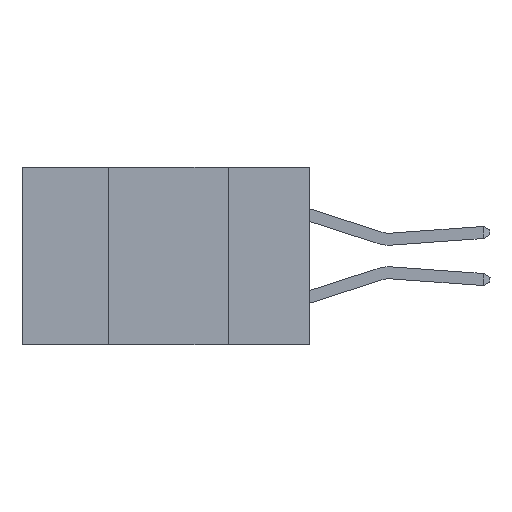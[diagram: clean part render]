
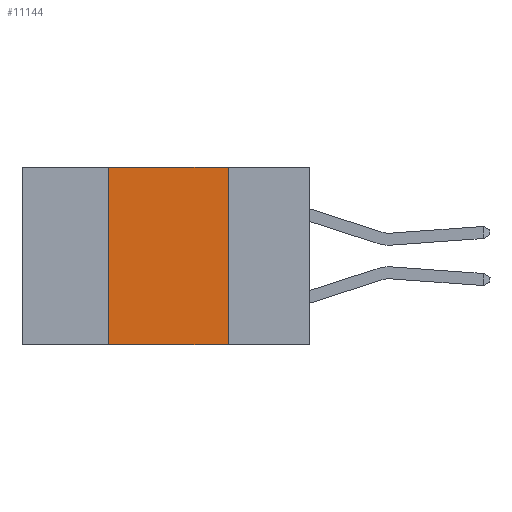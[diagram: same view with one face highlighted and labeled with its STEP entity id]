
A CAD part, left-side view. The second image highlights one B-rep face of the part: STEP entity #11144.
In plain terms, the highlighted planar face has unit normal (-1, 0, 0).
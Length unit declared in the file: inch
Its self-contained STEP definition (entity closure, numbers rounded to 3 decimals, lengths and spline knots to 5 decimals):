
#78 = VECTOR ( 'NONE', #6841, 39.37008 ) ;
#605 = CARTESIAN_POINT ( 'NONE',  ( 0., 0.17, 0. ) ) ;
#1331 = DIRECTION ( 'NONE',  ( 0., -1., 0. ) ) ;
#1500 = VERTEX_POINT ( 'NONE', #13177 ) ;
#1676 = LINE ( 'NONE', #15825, #78 ) ;
#2195 = CARTESIAN_POINT ( 'NONE',  ( 0., 0.6, 0. ) ) ;
#3289 = VERTEX_POINT ( 'NONE', #6100 ) ;
#3583 = VERTEX_POINT ( 'NONE', #18654 ) ;
#3704 = AXIS2_PLACEMENT_3D ( 'NONE', #2195, #12741, #5280 ) ;
#4783 = VERTEX_POINT ( 'NONE', #6198 ) ;
#5280 = DIRECTION ( 'NONE',  ( 0., 0., -1. ) ) ;
#6100 = CARTESIAN_POINT ( 'NONE',  ( 0., 0.17, 0. ) ) ;
#6198 = CARTESIAN_POINT ( 'NONE',  ( 0., 0.17, -0.37 ) ) ;
#6601 = EDGE_LOOP ( 'NONE', ( #7030, #7956, #11015, #7179 ) ) ;
#6708 = VECTOR ( 'NONE', #1331, 39.37008 ) ;
#6841 = DIRECTION ( 'NONE',  ( 0., -1., 0. ) ) ;
#6898 = PLANE ( 'NONE',  #3704 ) ;
#7030 = ORIENTED_EDGE ( 'NONE', *, *, #7323, .F. ) ;
#7179 = ORIENTED_EDGE ( 'NONE', *, *, #17079, .T. ) ;
#7323 = EDGE_CURVE ( 'NONE', #3289, #4783, #9662, .T. ) ;
#7956 = ORIENTED_EDGE ( 'NONE', *, *, #13563, .F. ) ;
#9662 = LINE ( 'NONE', #605, #12944 ) ;
#11015 = ORIENTED_EDGE ( 'NONE', *, *, #13642, .F. ) ;
#11074 = DIRECTION ( 'NONE',  ( 0., 0., -1. ) ) ;
#11144 = ADVANCED_FACE ( 'NONE', ( #18810 ), #6898, .F. ) ;
#11556 = CARTESIAN_POINT ( 'NONE',  ( 0., 0.42, 0. ) ) ;
#12741 = DIRECTION ( 'NONE',  ( 1., 0., 0. ) ) ;
#12944 = VECTOR ( 'NONE', #11074, 39.37008 ) ;
#13177 = CARTESIAN_POINT ( 'NONE',  ( 0., 0.42, 0. ) ) ;
#13563 = EDGE_CURVE ( 'NONE', #1500, #3289, #1676, .T. ) ;
#13642 = EDGE_CURVE ( 'NONE', #3583, #1500, #14933, .T. ) ;
#14933 = LINE ( 'NONE', #11556, #18398 ) ;
#15825 = CARTESIAN_POINT ( 'NONE',  ( 0., 0.6, 0. ) ) ;
#15863 = DIRECTION ( 'NONE',  ( 0., 0., 1. ) ) ;
#16328 = CARTESIAN_POINT ( 'NONE',  ( 0., 0.6, -0.37 ) ) ;
#17079 = EDGE_CURVE ( 'NONE', #3583, #4783, #18528, .T. ) ;
#18398 = VECTOR ( 'NONE', #15863, 39.37008 ) ;
#18528 = LINE ( 'NONE', #16328, #6708 ) ;
#18654 = CARTESIAN_POINT ( 'NONE',  ( 0., 0.42, -0.37 ) ) ;
#18810 = FACE_OUTER_BOUND ( 'NONE', #6601, .T. ) ;
